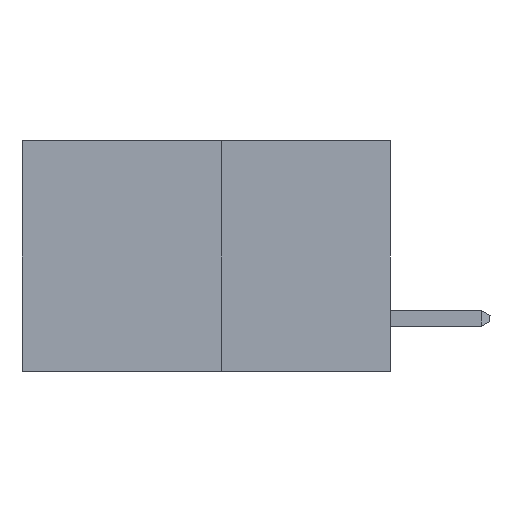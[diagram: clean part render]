
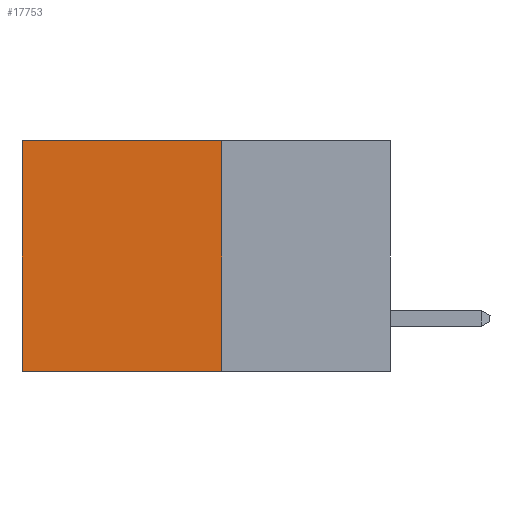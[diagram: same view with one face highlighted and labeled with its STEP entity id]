
A CAD part, left-side view. The second image highlights one B-rep face of the part: STEP entity #17753.
In plain terms, the highlighted planar face has unit normal (-1, 0, 0).
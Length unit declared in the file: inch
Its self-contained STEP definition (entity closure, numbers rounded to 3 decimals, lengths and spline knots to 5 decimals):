
#508 = EDGE_CURVE ( 'NONE', #6507, #16268, #17682, .T. ) ;
#990 = EDGE_CURVE ( 'NONE', #1796, #16322, #14578, .T. ) ;
#1112 = ORIENTED_EDGE ( 'NONE', *, *, #508, .F. ) ;
#1287 = ORIENTED_EDGE ( 'NONE', *, *, #9748, .T. ) ;
#1402 = CARTESIAN_POINT ( 'NONE',  ( 0.277, 0.27, -0.37 ) ) ;
#1796 = VERTEX_POINT ( 'NONE', #9918 ) ;
#2633 = DIRECTION ( 'NONE',  ( 0., 0., -1. ) ) ;
#3030 = EDGE_CURVE ( 'NONE', #16268, #16322, #8757, .T. ) ;
#3407 = VECTOR ( 'NONE', #11585, 39.37008 ) ;
#3425 = EDGE_LOOP ( 'NONE', ( #7409, #10528, #1112, #1287 ) ) ;
#3735 = CARTESIAN_POINT ( 'NONE',  ( 0.277, 0.27, 0. ) ) ;
#3806 = DIRECTION ( 'NONE',  ( 0., 1., 0. ) ) ;
#3945 = CARTESIAN_POINT ( 'NONE',  ( 0.277, 0.27, 0. ) ) ;
#4408 = CARTESIAN_POINT ( 'NONE',  ( 0.277, 0.59, -0.37 ) ) ;
#5789 = CARTESIAN_POINT ( 'NONE',  ( 0.277, 0.59, -0.37 ) ) ;
#6507 = VERTEX_POINT ( 'NONE', #3735 ) ;
#7122 = DIRECTION ( 'NONE',  ( 1., 0., 0. ) ) ;
#7409 = ORIENTED_EDGE ( 'NONE', *, *, #990, .T. ) ;
#7746 = CARTESIAN_POINT ( 'NONE',  ( 0.277, 0.27, -0.37 ) ) ;
#7951 = LINE ( 'NONE', #3945, #11248 ) ;
#8757 = LINE ( 'NONE', #7746, #15554 ) ;
#9262 = CARTESIAN_POINT ( 'NONE',  ( 0.277, 0.27, -0.37 ) ) ;
#9748 = EDGE_CURVE ( 'NONE', #6507, #1796, #7951, .T. ) ;
#9918 = CARTESIAN_POINT ( 'NONE',  ( 0.277, 0.59, 0. ) ) ;
#10528 = ORIENTED_EDGE ( 'NONE', *, *, #3030, .F. ) ;
#10782 = DIRECTION ( 'NONE',  ( 0., 1., 0. ) ) ;
#11001 = AXIS2_PLACEMENT_3D ( 'NONE', #1402, #7122, #16673 ) ;
#11248 = VECTOR ( 'NONE', #3806, 39.37008 ) ;
#11585 = DIRECTION ( 'NONE',  ( 0., 0., -1. ) ) ;
#12217 = FACE_OUTER_BOUND ( 'NONE', #3425, .T. ) ;
#13764 = VECTOR ( 'NONE', #2633, 39.37008 ) ;
#14578 = LINE ( 'NONE', #5789, #3407 ) ;
#15348 = CARTESIAN_POINT ( 'NONE',  ( 0.277, 0.27, -0.37 ) ) ;
#15362 = PLANE ( 'NONE',  #11001 ) ;
#15554 = VECTOR ( 'NONE', #10782, 39.37008 ) ;
#16268 = VERTEX_POINT ( 'NONE', #15348 ) ;
#16322 = VERTEX_POINT ( 'NONE', #4408 ) ;
#16673 = DIRECTION ( 'NONE',  ( 0., 0., -1. ) ) ;
#17682 = LINE ( 'NONE', #9262, #13764 ) ;
#17753 = ADVANCED_FACE ( 'NONE', ( #12217 ), #15362, .F. ) ;
